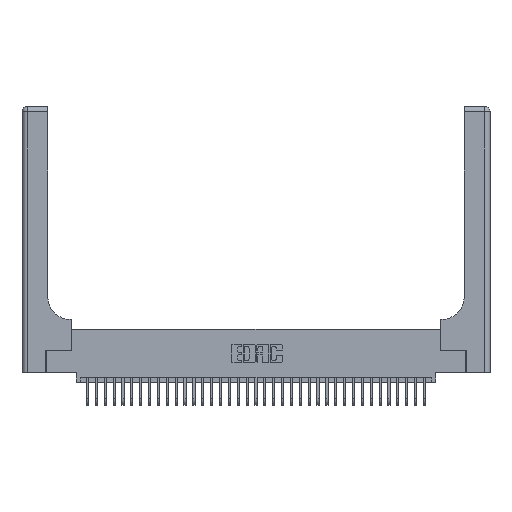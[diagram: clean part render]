
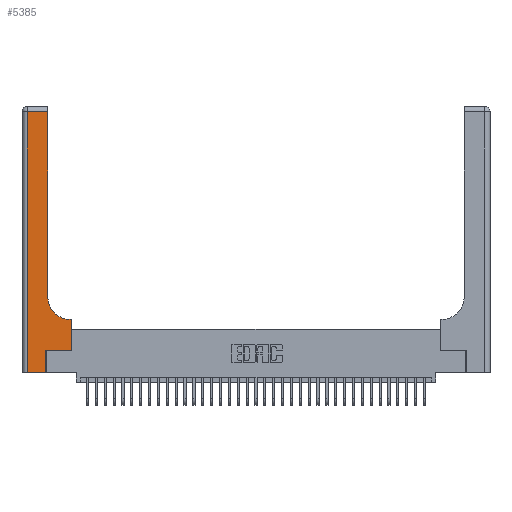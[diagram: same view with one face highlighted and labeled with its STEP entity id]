
A CAD part, top view. The second image highlights one B-rep face of the part: STEP entity #5385.
In plain terms, the highlighted planar face has unit normal (0, 0, 1).
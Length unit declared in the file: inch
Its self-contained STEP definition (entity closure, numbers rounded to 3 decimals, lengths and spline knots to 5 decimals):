
#192 = EDGE_CURVE ( 'NONE', #27740, #9677, #23555, .T. ) ;
#771 = LINE ( 'NONE', #33415, #15570 ) ;
#969 = ORIENTED_EDGE ( 'NONE', *, *, #10465, .T. ) ;
#1029 = DIRECTION ( 'NONE',  ( -1., 0., 0. ) ) ;
#1613 = AXIS2_PLACEMENT_3D ( 'NONE', #4242, #24784, #7192 ) ;
#1883 = ORIENTED_EDGE ( 'NONE', *, *, #10691, .T. ) ;
#2302 = DIRECTION ( 'NONE',  ( 0., 0., -1. ) ) ;
#3264 = DIRECTION ( 'NONE',  ( 0., -1., 0. ) ) ;
#3967 = AXIS2_PLACEMENT_3D ( 'NONE', #19964, #2302, #22902 ) ;
#4148 = ORIENTED_EDGE ( 'NONE', *, *, #22565, .T. ) ;
#4242 = CARTESIAN_POINT ( 'NONE',  ( 0.5415, 0.85, 0.37 ) ) ;
#5385 = ADVANCED_FACE ( 'NONE', ( #35529 ), #34476, .F. ) ;
#6961 = VECTOR ( 'NONE', #32077, 39.37008 ) ;
#7032 = CARTESIAN_POINT ( 'NONE',  ( 0.2915, 0.85, 0.37 ) ) ;
#7192 = DIRECTION ( 'NONE',  ( 1., 0., 0. ) ) ;
#8142 = VECTOR ( 'NONE', #13996, 39.37008 ) ;
#9677 = VERTEX_POINT ( 'NONE', #17718 ) ;
#9810 = EDGE_CURVE ( 'NONE', #33391, #11207, #18352, .T. ) ;
#10465 = EDGE_CURVE ( 'NONE', #16079, #17174, #771, .T. ) ;
#10691 = EDGE_CURVE ( 'NONE', #9677, #22453, #32467, .T. ) ;
#11132 = CARTESIAN_POINT ( 'NONE',  ( 0.269, 0.25, 0.37 ) ) ;
#11207 = VERTEX_POINT ( 'NONE', #16019 ) ;
#11426 = EDGE_LOOP ( 'NONE', ( #14133, #1883, #4148, #23098, #36754, #17916, #969, #31745, #28673 ) ) ;
#12980 = DIRECTION ( 'NONE',  ( 0., 1., 0. ) ) ;
#13904 = LINE ( 'NONE', #24575, #36288 ) ;
#13996 = DIRECTION ( 'NONE',  ( -1., 0., 0. ) ) ;
#14133 = ORIENTED_EDGE ( 'NONE', *, *, #192, .T. ) ;
#14179 = CARTESIAN_POINT ( 'NONE',  ( 0.06, 0., 0.37 ) ) ;
#15500 = DIRECTION ( 'NONE',  ( 1., 0., 0. ) ) ;
#15570 = VECTOR ( 'NONE', #12980, 39.37008 ) ;
#16019 = CARTESIAN_POINT ( 'NONE',  ( 0.269, 0., 0.37 ) ) ;
#16079 = VERTEX_POINT ( 'NONE', #34730 ) ;
#17174 = VERTEX_POINT ( 'NONE', #24786 ) ;
#17718 = CARTESIAN_POINT ( 'NONE',  ( 0.2915, 2.94, 0.37 ) ) ;
#17916 = ORIENTED_EDGE ( 'NONE', *, *, #30395, .T. ) ;
#18352 = LINE ( 'NONE', #32991, #19293 ) ;
#18772 = DIRECTION ( 'NONE',  ( 0., 1., 0. ) ) ;
#19227 = EDGE_CURVE ( 'NONE', #11207, #27987, #28844, .T. ) ;
#19293 = VECTOR ( 'NONE', #15500, 39.37008 ) ;
#19964 = CARTESIAN_POINT ( 'NONE',  ( 0., 3., 0.37 ) ) ;
#20094 = CIRCLE ( 'NONE', #1613, 0.25 ) ;
#22013 = VECTOR ( 'NONE', #18772, 39.37008 ) ;
#22453 = VERTEX_POINT ( 'NONE', #34789 ) ;
#22565 = EDGE_CURVE ( 'NONE', #22453, #33391, #26292, .T. ) ;
#22735 = EDGE_CURVE ( 'NONE', #17174, #32317, #13904, .T. ) ;
#22902 = DIRECTION ( 'NONE',  ( -1., 0., 0. ) ) ;
#23098 = ORIENTED_EDGE ( 'NONE', *, *, #9810, .T. ) ;
#23555 = LINE ( 'NONE', #29167, #6961 ) ;
#24111 = LINE ( 'NONE', #11132, #25019 ) ;
#24575 = CARTESIAN_POINT ( 'NONE',  ( 0.2915, 0.6, 0.37 ) ) ;
#24784 = DIRECTION ( 'NONE',  ( 0., 0., -1. ) ) ;
#24786 = CARTESIAN_POINT ( 'NONE',  ( 0.5585, 0.6, 0.37 ) ) ;
#25019 = VECTOR ( 'NONE', #34912, 39.37008 ) ;
#26292 = LINE ( 'NONE', #29562, #34018 ) ;
#27740 = VERTEX_POINT ( 'NONE', #7032 ) ;
#27987 = VERTEX_POINT ( 'NONE', #34302 ) ;
#28208 = CARTESIAN_POINT ( 'NONE',  ( 0.5415, 0.6, 0.37 ) ) ;
#28571 = CARTESIAN_POINT ( 'NONE',  ( 0., 2.94, 0.37 ) ) ;
#28673 = ORIENTED_EDGE ( 'NONE', *, *, #37532, .T. ) ;
#28844 = LINE ( 'NONE', #36248, #22013 ) ;
#29167 = CARTESIAN_POINT ( 'NONE',  ( 0.2915, 3., 0.37 ) ) ;
#29562 = CARTESIAN_POINT ( 'NONE',  ( 0.06, 3., 0.37 ) ) ;
#30395 = EDGE_CURVE ( 'NONE', #27987, #16079, #24111, .T. ) ;
#31745 = ORIENTED_EDGE ( 'NONE', *, *, #22735, .T. ) ;
#32077 = DIRECTION ( 'NONE',  ( 0., 1., 0. ) ) ;
#32317 = VERTEX_POINT ( 'NONE', #28208 ) ;
#32467 = LINE ( 'NONE', #28571, #8142 ) ;
#32991 = CARTESIAN_POINT ( 'NONE',  ( 0., 0., 0.37 ) ) ;
#33391 = VERTEX_POINT ( 'NONE', #14179 ) ;
#33415 = CARTESIAN_POINT ( 'NONE',  ( 0.5585, 0.25, 0.37 ) ) ;
#34018 = VECTOR ( 'NONE', #3264, 39.37008 ) ;
#34302 = CARTESIAN_POINT ( 'NONE',  ( 0.269, 0.25, 0.37 ) ) ;
#34476 = PLANE ( 'NONE',  #3967 ) ;
#34730 = CARTESIAN_POINT ( 'NONE',  ( 0.5585, 0.25, 0.37 ) ) ;
#34789 = CARTESIAN_POINT ( 'NONE',  ( 0.06, 2.94, 0.37 ) ) ;
#34912 = DIRECTION ( 'NONE',  ( 1., 0., 0. ) ) ;
#35529 = FACE_OUTER_BOUND ( 'NONE', #11426, .T. ) ;
#36248 = CARTESIAN_POINT ( 'NONE',  ( 0.269, 0., 0.37 ) ) ;
#36288 = VECTOR ( 'NONE', #1029, 39.37008 ) ;
#36754 = ORIENTED_EDGE ( 'NONE', *, *, #19227, .T. ) ;
#37532 = EDGE_CURVE ( 'NONE', #32317, #27740, #20094, .T. ) ;
